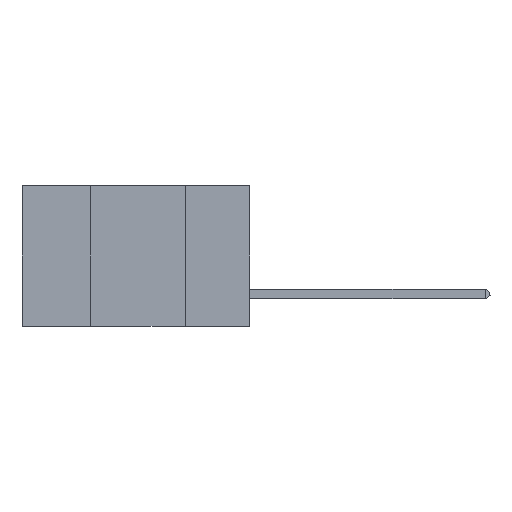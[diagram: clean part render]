
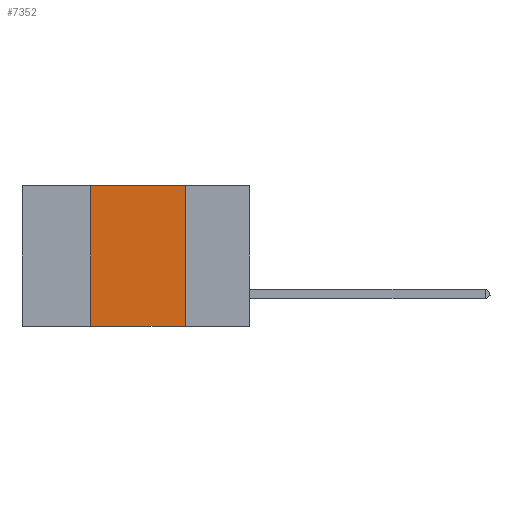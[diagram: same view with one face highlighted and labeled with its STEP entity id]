
A CAD part, left-side view. The second image highlights one B-rep face of the part: STEP entity #7352.
In plain terms, the highlighted planar face has unit normal (-1, 0, 0).
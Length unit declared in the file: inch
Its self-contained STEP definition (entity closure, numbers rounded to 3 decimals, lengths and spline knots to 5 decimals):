
#152 = CARTESIAN_POINT ( 'NONE',  ( 0., 0.42, 0. ) ) ;
#388 = DIRECTION ( 'NONE',  ( 0., 0., -1. ) ) ;
#892 = AXIS2_PLACEMENT_3D ( 'NONE', #8161, #4610, #388 ) ;
#1039 = DIRECTION ( 'NONE',  ( 0., 0., 1. ) ) ;
#1128 = VERTEX_POINT ( 'NONE', #152 ) ;
#1182 = DIRECTION ( 'NONE',  ( 0., -1., 0. ) ) ;
#2591 = CARTESIAN_POINT ( 'NONE',  ( 0., 0.6, -0.37 ) ) ;
#2699 = EDGE_CURVE ( 'NONE', #8103, #1128, #10340, .T. ) ;
#2724 = CARTESIAN_POINT ( 'NONE',  ( 0., 0.17, -0.37 ) ) ;
#2919 = CARTESIAN_POINT ( 'NONE',  ( 0., 0.42, -0.37 ) ) ;
#3797 = CARTESIAN_POINT ( 'NONE',  ( 0., 0.17, 0. ) ) ;
#4359 = VECTOR ( 'NONE', #1182, 39.37008 ) ;
#4413 = EDGE_CURVE ( 'NONE', #8103, #10916, #10838, .T. ) ;
#4574 = ORIENTED_EDGE ( 'NONE', *, *, #5938, .F. ) ;
#4610 = DIRECTION ( 'NONE',  ( 1., 0., 0. ) ) ;
#5431 = ORIENTED_EDGE ( 'NONE', *, *, #2699, .F. ) ;
#5938 = EDGE_CURVE ( 'NONE', #6069, #10916, #7517, .T. ) ;
#5976 = VECTOR ( 'NONE', #1039, 39.37008 ) ;
#6069 = VERTEX_POINT ( 'NONE', #3797 ) ;
#6282 = CARTESIAN_POINT ( 'NONE',  ( 0., 0.42, 0. ) ) ;
#6338 = VECTOR ( 'NONE', #9584, 39.37008 ) ;
#6416 = PLANE ( 'NONE',  #892 ) ;
#7244 = FACE_OUTER_BOUND ( 'NONE', #11166, .T. ) ;
#7352 = ADVANCED_FACE ( 'NONE', ( #7244 ), #6416, .F. ) ;
#7387 = VECTOR ( 'NONE', #9190, 39.37008 ) ;
#7517 = LINE ( 'NONE', #10834, #7387 ) ;
#7759 = LINE ( 'NONE', #9130, #4359 ) ;
#7762 = ORIENTED_EDGE ( 'NONE', *, *, #4413, .T. ) ;
#8103 = VERTEX_POINT ( 'NONE', #2919 ) ;
#8161 = CARTESIAN_POINT ( 'NONE',  ( 0., 0.6, 0. ) ) ;
#9130 = CARTESIAN_POINT ( 'NONE',  ( 0., 0.6, 0. ) ) ;
#9190 = DIRECTION ( 'NONE',  ( 0., 0., -1. ) ) ;
#9584 = DIRECTION ( 'NONE',  ( 0., -1., 0. ) ) ;
#9691 = ORIENTED_EDGE ( 'NONE', *, *, #9909, .F. ) ;
#9909 = EDGE_CURVE ( 'NONE', #1128, #6069, #7759, .T. ) ;
#10340 = LINE ( 'NONE', #6282, #5976 ) ;
#10834 = CARTESIAN_POINT ( 'NONE',  ( 0., 0.17, 0. ) ) ;
#10838 = LINE ( 'NONE', #2591, #6338 ) ;
#10916 = VERTEX_POINT ( 'NONE', #2724 ) ;
#11166 = EDGE_LOOP ( 'NONE', ( #4574, #9691, #5431, #7762 ) ) ;
